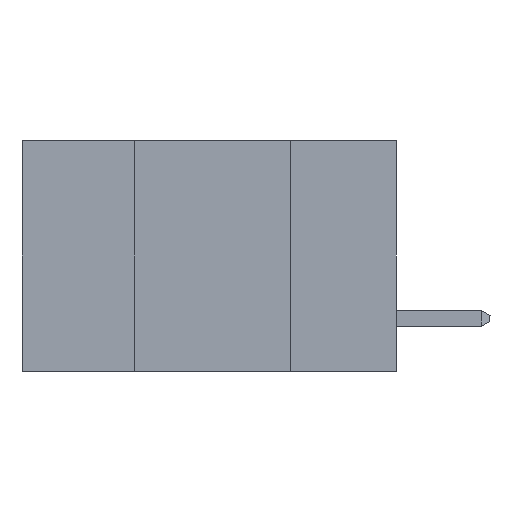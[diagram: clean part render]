
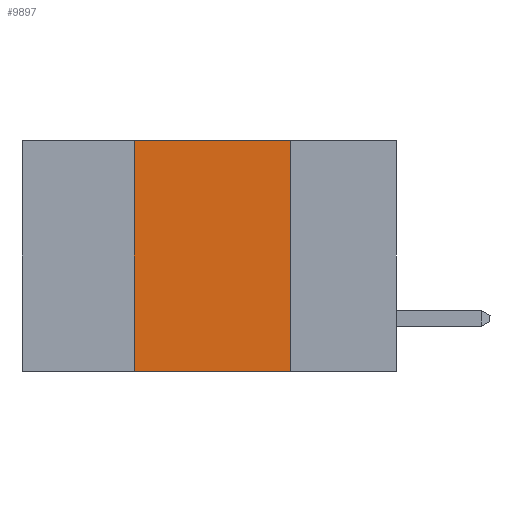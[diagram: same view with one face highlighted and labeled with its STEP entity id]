
A CAD part, left-side view. The second image highlights one B-rep face of the part: STEP entity #9897.
In plain terms, the highlighted planar face has unit normal (-1, 0, 0).
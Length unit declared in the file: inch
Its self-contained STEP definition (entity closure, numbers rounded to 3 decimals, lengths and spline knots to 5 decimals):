
#106 = LINE ( 'NONE', #3036, #19747 ) ;
#733 = VERTEX_POINT ( 'NONE', #16120 ) ;
#944 = PLANE ( 'NONE',  #8356 ) ;
#1605 = EDGE_CURVE ( 'NONE', #16224, #1957, #13586, .T. ) ;
#1957 = VERTEX_POINT ( 'NONE', #3823 ) ;
#2186 = EDGE_LOOP ( 'NONE', ( #19921, #10033, #13476, #3579 ) ) ;
#2932 = DIRECTION ( 'NONE',  ( 0., 0., -1. ) ) ;
#2956 = CARTESIAN_POINT ( 'NONE',  ( 0., 0.42, -0.37 ) ) ;
#3036 = CARTESIAN_POINT ( 'NONE',  ( 0., 0.17, -0.37 ) ) ;
#3579 = ORIENTED_EDGE ( 'NONE', *, *, #1605, .T. ) ;
#3823 = CARTESIAN_POINT ( 'NONE',  ( 0., 0.17, -0.37 ) ) ;
#4281 = DIRECTION ( 'NONE',  ( 0., 0., -1. ) ) ;
#6093 = VECTOR ( 'NONE', #11832, 39.37008 ) ;
#6247 = LINE ( 'NONE', #2956, #6446 ) ;
#6440 = DIRECTION ( 'NONE',  ( 0., 0., 1. ) ) ;
#6446 = VECTOR ( 'NONE', #6440, 39.37008 ) ;
#7169 = CARTESIAN_POINT ( 'NONE',  ( 0., 0.6, 0. ) ) ;
#8356 = AXIS2_PLACEMENT_3D ( 'NONE', #7169, #13333, #4281 ) ;
#8905 = VERTEX_POINT ( 'NONE', #19199 ) ;
#9897 = ADVANCED_FACE ( 'NONE', ( #13436 ), #944, .F. ) ;
#10033 = ORIENTED_EDGE ( 'NONE', *, *, #10842, .F. ) ;
#10527 = LINE ( 'NONE', #12215, #6093 ) ;
#10842 = EDGE_CURVE ( 'NONE', #733, #8905, #10527, .T. ) ;
#11391 = EDGE_CURVE ( 'NONE', #16224, #733, #6247, .T. ) ;
#11764 = EDGE_CURVE ( 'NONE', #8905, #1957, #106, .T. ) ;
#11832 = DIRECTION ( 'NONE',  ( 0., -1., 0. ) ) ;
#12215 = CARTESIAN_POINT ( 'NONE',  ( 0., 0.6, 0. ) ) ;
#13333 = DIRECTION ( 'NONE',  ( 1., 0., 0. ) ) ;
#13436 = FACE_OUTER_BOUND ( 'NONE', #2186, .T. ) ;
#13476 = ORIENTED_EDGE ( 'NONE', *, *, #11391, .F. ) ;
#13586 = LINE ( 'NONE', #15428, #17393 ) ;
#15428 = CARTESIAN_POINT ( 'NONE',  ( 0., 0.6, -0.37 ) ) ;
#16120 = CARTESIAN_POINT ( 'NONE',  ( 0., 0.42, 0. ) ) ;
#16224 = VERTEX_POINT ( 'NONE', #17492 ) ;
#17057 = DIRECTION ( 'NONE',  ( 0., -1., 0. ) ) ;
#17393 = VECTOR ( 'NONE', #17057, 39.37008 ) ;
#17492 = CARTESIAN_POINT ( 'NONE',  ( 0., 0.42, -0.37 ) ) ;
#19199 = CARTESIAN_POINT ( 'NONE',  ( 0., 0.17, 0. ) ) ;
#19747 = VECTOR ( 'NONE', #2932, 39.37008 ) ;
#19921 = ORIENTED_EDGE ( 'NONE', *, *, #11764, .F. ) ;
